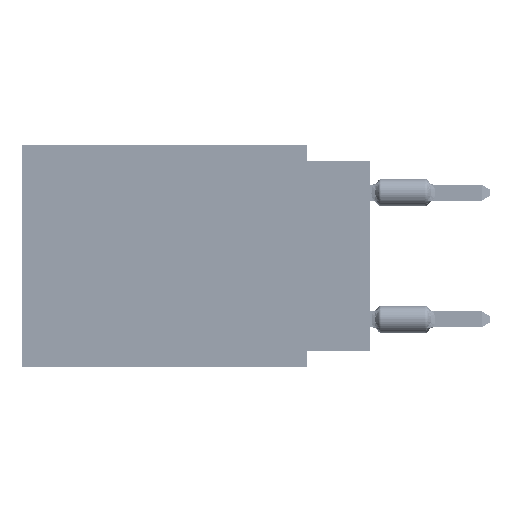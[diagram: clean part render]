
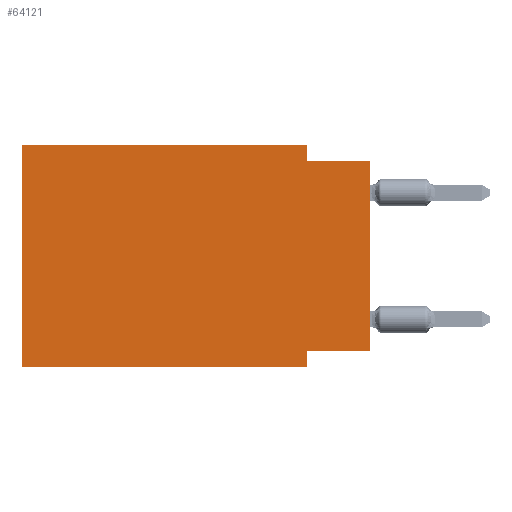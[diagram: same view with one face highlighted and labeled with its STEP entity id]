
A CAD part, left-side view. The second image highlights one B-rep face of the part: STEP entity #64121.
In plain terms, the highlighted planar face has unit normal (-1, 0, 0).
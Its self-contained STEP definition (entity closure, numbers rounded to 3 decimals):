
#602 = LINE ( 'NONE', #21942, #52855 ) ;
#1087 = DIRECTION ( 'NONE',  ( 0., 0., -1. ) ) ;
#1723 = CARTESIAN_POINT ( 'NONE',  ( 0., 0., -0.635 ) ) ;
#2401 = EDGE_CURVE ( 'NONE', #48236, #9421, #5198, .T. ) ;
#5088 = EDGE_CURVE ( 'NONE', #9421, #28914, #10746, .T. ) ;
#5198 = LINE ( 'NONE', #47852, #31014 ) ;
#6244 = CARTESIAN_POINT ( 'NONE',  ( 0., 13.97, -8.89 ) ) ;
#6414 = EDGE_CURVE ( 'NONE', #43153, #28914, #53795, .T. ) ;
#6606 = EDGE_LOOP ( 'NONE', ( #43006, #21400, #48917, #33619, #15582, #66114, #27290, #36816 ) ) ;
#6701 = PLANE ( 'NONE',  #12728 ) ;
#7737 = FACE_OUTER_BOUND ( 'NONE', #6606, .T. ) ;
#8749 = EDGE_CURVE ( 'NONE', #43153, #21510, #17230, .T. ) ;
#9381 = LINE ( 'NONE', #40865, #34288 ) ;
#9421 = VERTEX_POINT ( 'NONE', #47481 ) ;
#10354 = CARTESIAN_POINT ( 'NONE',  ( 0., 2.54, -0.635 ) ) ;
#10746 = LINE ( 'NONE', #22296, #15512 ) ;
#12728 = AXIS2_PLACEMENT_3D ( 'NONE', #22805, #39573, #1087 ) ;
#13817 = VECTOR ( 'NONE', #17472, 1000. ) ;
#13879 = VERTEX_POINT ( 'NONE', #64903 ) ;
#15512 = VECTOR ( 'NONE', #43627, 1000. ) ;
#15582 = ORIENTED_EDGE ( 'NONE', *, *, #8749, .F. ) ;
#16046 = CARTESIAN_POINT ( 'NONE',  ( 0., 2.54, -8.89 ) ) ;
#16876 = VECTOR ( 'NONE', #42940, 1000. ) ;
#17230 = LINE ( 'NONE', #34329, #42676 ) ;
#17472 = DIRECTION ( 'NONE',  ( 0., -1., 0. ) ) ;
#21250 = VECTOR ( 'NONE', #48551, 1000. ) ;
#21258 = EDGE_CURVE ( 'NONE', #36746, #46272, #22362, .T. ) ;
#21400 = ORIENTED_EDGE ( 'NONE', *, *, #21258, .F. ) ;
#21510 = VERTEX_POINT ( 'NONE', #62912 ) ;
#21942 = CARTESIAN_POINT ( 'NONE',  ( 0., 0., 0. ) ) ;
#22296 = CARTESIAN_POINT ( 'NONE',  ( 0., 2.54, -8.89 ) ) ;
#22362 = LINE ( 'NONE', #1723, #13817 ) ;
#22805 = CARTESIAN_POINT ( 'NONE',  ( 0., 13.97, 0. ) ) ;
#23656 = EDGE_CURVE ( 'NONE', #13879, #36746, #9381, .T. ) ;
#25428 = DIRECTION ( 'NONE',  ( 0., 0., -1. ) ) ;
#27290 = ORIENTED_EDGE ( 'NONE', *, *, #5088, .F. ) ;
#28914 = VERTEX_POINT ( 'NONE', #16046 ) ;
#31014 = VECTOR ( 'NONE', #64010, 1000. ) ;
#31900 = CARTESIAN_POINT ( 'NONE',  ( 0., 0., -0.635 ) ) ;
#32050 = CARTESIAN_POINT ( 'NONE',  ( 0., 13.97, 0. ) ) ;
#33469 = LINE ( 'NONE', #32050, #16876 ) ;
#33619 = ORIENTED_EDGE ( 'NONE', *, *, #68505, .F. ) ;
#34288 = VECTOR ( 'NONE', #25428, 1000. ) ;
#34329 = CARTESIAN_POINT ( 'NONE',  ( 0., 13.97, 0. ) ) ;
#36746 = VERTEX_POINT ( 'NONE', #10354 ) ;
#36816 = ORIENTED_EDGE ( 'NONE', *, *, #2401, .F. ) ;
#39537 = CARTESIAN_POINT ( 'NONE',  ( 0., 13.97, -8.89 ) ) ;
#39573 = DIRECTION ( 'NONE',  ( 1., 0., 0. ) ) ;
#40865 = CARTESIAN_POINT ( 'NONE',  ( 0., 2.54, 0. ) ) ;
#42676 = VECTOR ( 'NONE', #66230, 1000. ) ;
#42918 = DIRECTION ( 'NONE',  ( 0., 0., 1. ) ) ;
#42940 = DIRECTION ( 'NONE',  ( 0., -1., 0. ) ) ;
#43006 = ORIENTED_EDGE ( 'NONE', *, *, #57885, .T. ) ;
#43153 = VERTEX_POINT ( 'NONE', #39537 ) ;
#43627 = DIRECTION ( 'NONE',  ( 0., 0., -1. ) ) ;
#46272 = VERTEX_POINT ( 'NONE', #31900 ) ;
#47481 = CARTESIAN_POINT ( 'NONE',  ( 0., 2.54, -8.255 ) ) ;
#47852 = CARTESIAN_POINT ( 'NONE',  ( 0., 0., -8.255 ) ) ;
#48236 = VERTEX_POINT ( 'NONE', #62860 ) ;
#48551 = DIRECTION ( 'NONE',  ( 0., -1., 0. ) ) ;
#48917 = ORIENTED_EDGE ( 'NONE', *, *, #23656, .F. ) ;
#52855 = VECTOR ( 'NONE', #42918, 1000. ) ;
#53795 = LINE ( 'NONE', #6244, #21250 ) ;
#57885 = EDGE_CURVE ( 'NONE', #48236, #46272, #602, .T. ) ;
#62860 = CARTESIAN_POINT ( 'NONE',  ( 0., 0., -8.255 ) ) ;
#62912 = CARTESIAN_POINT ( 'NONE',  ( 0., 13.97, 0. ) ) ;
#64010 = DIRECTION ( 'NONE',  ( 0., 1., 0. ) ) ;
#64121 = ADVANCED_FACE ( 'NONE', ( #7737 ), #6701, .F. ) ;
#64903 = CARTESIAN_POINT ( 'NONE',  ( 0., 2.54, 0. ) ) ;
#66114 = ORIENTED_EDGE ( 'NONE', *, *, #6414, .T. ) ;
#66230 = DIRECTION ( 'NONE',  ( 0., 0., 1. ) ) ;
#68505 = EDGE_CURVE ( 'NONE', #21510, #13879, #33469, .T. ) ;
